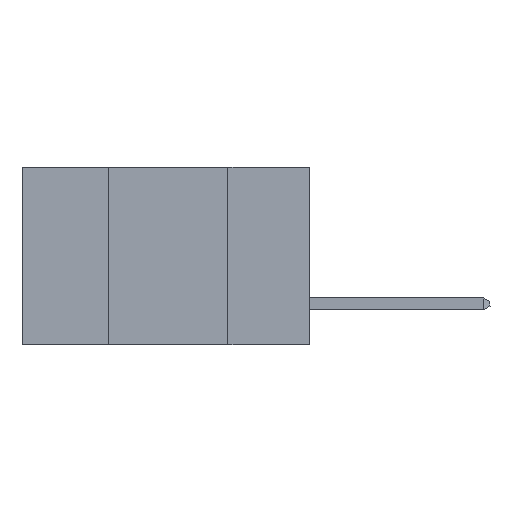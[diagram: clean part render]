
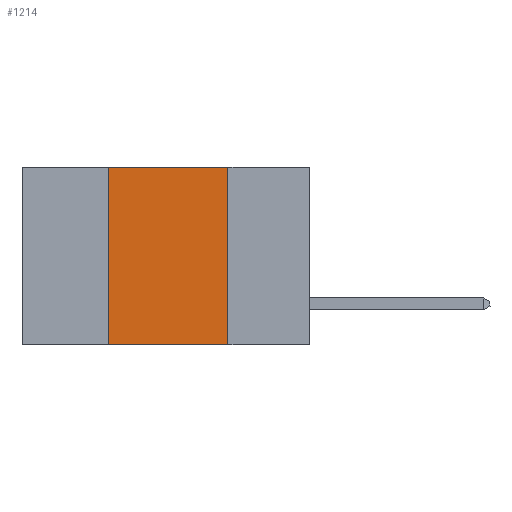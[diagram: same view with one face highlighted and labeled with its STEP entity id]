
A CAD part, left-side view. The second image highlights one B-rep face of the part: STEP entity #1214.
In plain terms, the highlighted planar face has unit normal (-1, 0, 0).
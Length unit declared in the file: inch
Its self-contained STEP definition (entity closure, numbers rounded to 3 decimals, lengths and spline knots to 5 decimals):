
#121 = CARTESIAN_POINT ( 'NONE',  ( 0., 0.17, 0. ) ) ;
#571 = CARTESIAN_POINT ( 'NONE',  ( 0., 0.6, -0.37 ) ) ;
#875 = VECTOR ( 'NONE', #3048, 39.37008 ) ;
#977 = VERTEX_POINT ( 'NONE', #7178 ) ;
#1214 = ADVANCED_FACE ( 'NONE', ( #9561 ), #5381, .F. ) ;
#1487 = LINE ( 'NONE', #571, #875 ) ;
#2364 = CARTESIAN_POINT ( 'NONE',  ( 0., 0.42, 0. ) ) ;
#2523 = AXIS2_PLACEMENT_3D ( 'NONE', #3644, #3779, #3793 ) ;
#2575 = CARTESIAN_POINT ( 'NONE',  ( 0., 0.42, -0.37 ) ) ;
#2592 = EDGE_CURVE ( 'NONE', #8240, #8491, #7824, .T. ) ;
#2903 = DIRECTION ( 'NONE',  ( 0., 0., -1. ) ) ;
#3048 = DIRECTION ( 'NONE',  ( 0., -1., 0. ) ) ;
#3123 = VERTEX_POINT ( 'NONE', #2575 ) ;
#3351 = CARTESIAN_POINT ( 'NONE',  ( 0., 0.17, 0. ) ) ;
#3460 = ORIENTED_EDGE ( 'NONE', *, *, #4402, .T. ) ;
#3644 = CARTESIAN_POINT ( 'NONE',  ( 0., 0.6, 0. ) ) ;
#3756 = ORIENTED_EDGE ( 'NONE', *, *, #2592, .F. ) ;
#3779 = DIRECTION ( 'NONE',  ( 1., 0., 0. ) ) ;
#3793 = DIRECTION ( 'NONE',  ( 0., 0., -1. ) ) ;
#4246 = ORIENTED_EDGE ( 'NONE', *, *, #4977, .F. ) ;
#4402 = EDGE_CURVE ( 'NONE', #3123, #8491, #1487, .T. ) ;
#4557 = LINE ( 'NONE', #2364, #8496 ) ;
#4584 = ORIENTED_EDGE ( 'NONE', *, *, #9317, .F. ) ;
#4977 = EDGE_CURVE ( 'NONE', #3123, #977, #4557, .T. ) ;
#5344 = DIRECTION ( 'NONE',  ( 0., 0., 1. ) ) ;
#5381 = PLANE ( 'NONE',  #2523 ) ;
#5928 = VECTOR ( 'NONE', #2903, 39.37008 ) ;
#6464 = CARTESIAN_POINT ( 'NONE',  ( 0., 0.6, 0. ) ) ;
#6880 = LINE ( 'NONE', #6464, #8640 ) ;
#7178 = CARTESIAN_POINT ( 'NONE',  ( 0., 0.42, 0. ) ) ;
#7650 = EDGE_LOOP ( 'NONE', ( #3756, #4584, #4246, #3460 ) ) ;
#7824 = LINE ( 'NONE', #3351, #5928 ) ;
#8240 = VERTEX_POINT ( 'NONE', #121 ) ;
#8491 = VERTEX_POINT ( 'NONE', #9236 ) ;
#8496 = VECTOR ( 'NONE', #5344, 39.37008 ) ;
#8640 = VECTOR ( 'NONE', #8671, 39.37008 ) ;
#8671 = DIRECTION ( 'NONE',  ( 0., -1., 0. ) ) ;
#9236 = CARTESIAN_POINT ( 'NONE',  ( 0., 0.17, -0.37 ) ) ;
#9317 = EDGE_CURVE ( 'NONE', #977, #8240, #6880, .T. ) ;
#9561 = FACE_OUTER_BOUND ( 'NONE', #7650, .T. ) ;
